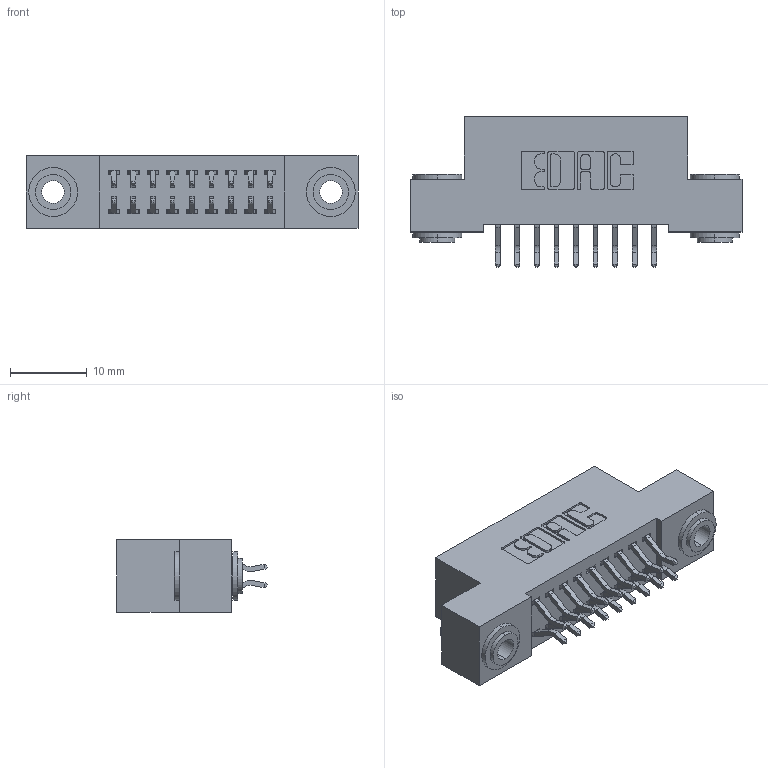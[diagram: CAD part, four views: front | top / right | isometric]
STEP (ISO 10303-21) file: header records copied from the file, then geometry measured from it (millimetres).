
FILE_DESCRIPTION (( 'STEP AP203' ), '1' );
FILE_NAME ('342-018-556-203.STEP', '2018-08-10T21:45:27', ( '' ), ( '' ), 'SwSTEP 2.0', 'SolidWorks 2016', '' );
FILE_SCHEMA (( 'CONFIG_CONTROL_DESIGN' ));
Length unit declared in the file: inch
Products named in the file (4): 342-018-556-203; 342 Part_.156 TH; 345-292-001_556 Tail; 342-250-002_345-250-002-102
Assembly tree (21 placements, depth 2):
  342-018-556-203
    342 Part_.156 TH
    345-292-001_556 Tail  x18
    342-250-002_345-250-002-102  x2
Bounding box: 43.18 x 19.58 x 9.4 mm (x, y, z)
Volume: 3745.9 mm3; surface area: 5480.8 mm2
Topology: 21 solids, 21 shells, 1192 faces, 3489 edges, 2298 vertices
Faces by surface type: plane 796, cylinder 388, cone 8
Entity records: 10796 total; most frequent: CARTESIAN_POINT 1817, ORIENTED_EDGE 1734, DIRECTION 1633, EDGE_CURVE 867, LINE 707, VECTOR 707, VERTEX_POINT 574, AXIS2_PLACEMENT_3D 463
